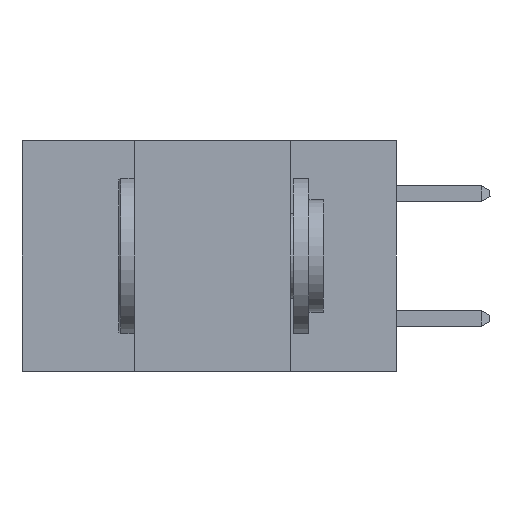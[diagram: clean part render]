
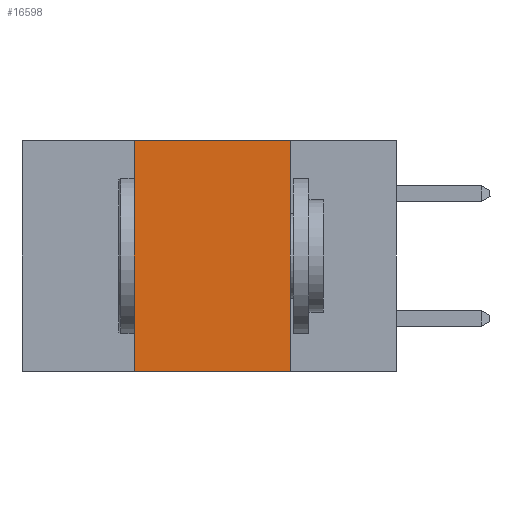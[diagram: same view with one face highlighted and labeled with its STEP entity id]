
A CAD part, left-side view. The second image highlights one B-rep face of the part: STEP entity #16598.
In plain terms, the highlighted planar face has unit normal (-1, 0, 0).
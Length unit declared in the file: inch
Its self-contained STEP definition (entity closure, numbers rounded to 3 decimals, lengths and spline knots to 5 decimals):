
#421 = CARTESIAN_POINT ( 'NONE',  ( 0., 0.17, 0. ) ) ;
#725 = CARTESIAN_POINT ( 'NONE',  ( 0., 0.17, 0. ) ) ;
#1778 = CARTESIAN_POINT ( 'NONE',  ( 0., 0.42, 0. ) ) ;
#2302 = VECTOR ( 'NONE', #10788, 39.37008 ) ;
#2571 = CARTESIAN_POINT ( 'NONE',  ( 0., 0.17, -0.37 ) ) ;
#2747 = VECTOR ( 'NONE', #5864, 39.37008 ) ;
#2907 = AXIS2_PLACEMENT_3D ( 'NONE', #9165, #4821, #9361 ) ;
#3140 = LINE ( 'NONE', #15906, #9851 ) ;
#4039 = EDGE_CURVE ( 'NONE', #18920, #4147, #14421, .T. ) ;
#4147 = VERTEX_POINT ( 'NONE', #14831 ) ;
#4284 = EDGE_CURVE ( 'NONE', #16790, #15803, #19048, .T. ) ;
#4821 = DIRECTION ( 'NONE',  ( 1., 0., 0. ) ) ;
#4952 = PLANE ( 'NONE',  #2907 ) ;
#5735 = CARTESIAN_POINT ( 'NONE',  ( 0., 0.6, -0.37 ) ) ;
#5864 = DIRECTION ( 'NONE',  ( 0., -1., 0. ) ) ;
#6131 = EDGE_CURVE ( 'NONE', #18920, #15803, #10660, .T. ) ;
#6610 = CARTESIAN_POINT ( 'NONE',  ( 0., 0.42, -0.37 ) ) ;
#7864 = ORIENTED_EDGE ( 'NONE', *, *, #4284, .F. ) ;
#8360 = DIRECTION ( 'NONE',  ( 0., -1., 0. ) ) ;
#8857 = VECTOR ( 'NONE', #15291, 39.37008 ) ;
#9165 = CARTESIAN_POINT ( 'NONE',  ( 0., 0.6, 0. ) ) ;
#9361 = DIRECTION ( 'NONE',  ( 0., 0., -1. ) ) ;
#9851 = VECTOR ( 'NONE', #8360, 39.37008 ) ;
#10262 = ORIENTED_EDGE ( 'NONE', *, *, #4039, .F. ) ;
#10660 = LINE ( 'NONE', #5735, #2747 ) ;
#10788 = DIRECTION ( 'NONE',  ( 0., 0., -1. ) ) ;
#12681 = EDGE_LOOP ( 'NONE', ( #7864, #15544, #10262, #14943 ) ) ;
#14421 = LINE ( 'NONE', #1778, #8857 ) ;
#14831 = CARTESIAN_POINT ( 'NONE',  ( 0., 0.42, 0. ) ) ;
#14943 = ORIENTED_EDGE ( 'NONE', *, *, #6131, .T. ) ;
#15291 = DIRECTION ( 'NONE',  ( 0., 0., 1. ) ) ;
#15544 = ORIENTED_EDGE ( 'NONE', *, *, #16838, .F. ) ;
#15803 = VERTEX_POINT ( 'NONE', #2571 ) ;
#15906 = CARTESIAN_POINT ( 'NONE',  ( 0., 0.6, 0. ) ) ;
#16566 = FACE_OUTER_BOUND ( 'NONE', #12681, .T. ) ;
#16598 = ADVANCED_FACE ( 'NONE', ( #16566 ), #4952, .F. ) ;
#16790 = VERTEX_POINT ( 'NONE', #725 ) ;
#16838 = EDGE_CURVE ( 'NONE', #4147, #16790, #3140, .T. ) ;
#18920 = VERTEX_POINT ( 'NONE', #6610 ) ;
#19048 = LINE ( 'NONE', #421, #2302 ) ;
